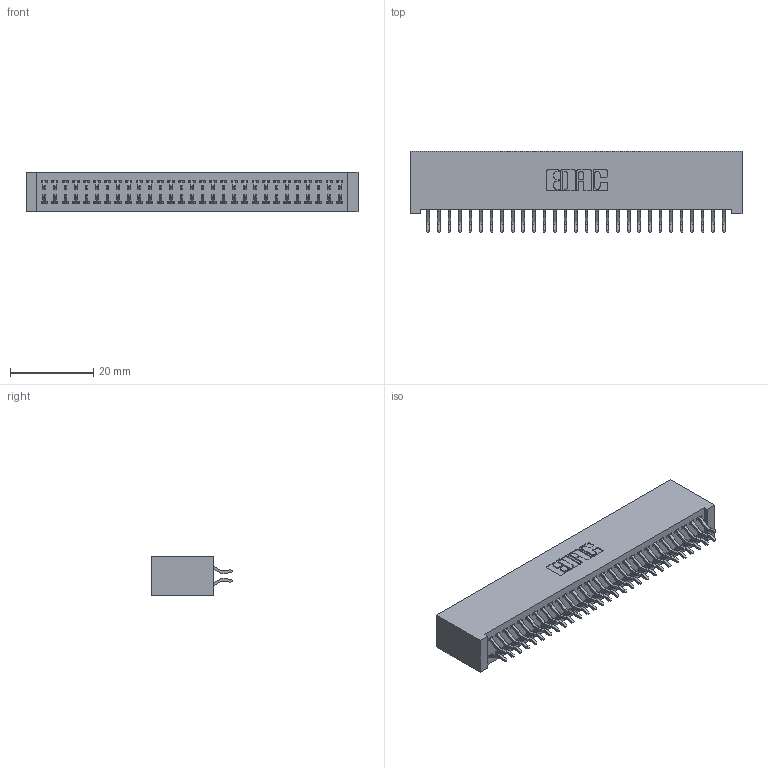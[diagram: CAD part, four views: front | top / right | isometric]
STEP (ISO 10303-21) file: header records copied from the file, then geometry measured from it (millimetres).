
FILE_DESCRIPTION (( 'STEP AP203' ), '1' );
FILE_NAME ('392-058-556-201.STEP', '2019-10-08T16:53:33', ( '' ), ( '' ), 'SwSTEP 2.0', 'SolidWorks 2016', '' );
FILE_SCHEMA (( 'CONFIG_CONTROL_DESIGN' ));
Length unit declared in the file: inch
Products named in the file (3): 392-058-556-201; 342 Part_Lugless; 345-292-001_556 Tail
Assembly tree (59 placements, depth 2):
  392-058-556-201
    342 Part_Lugless
    345-292-001_556 Tail  x58
Bounding box: 79.91 x 19.58 x 9.4 mm (x, y, z)
Volume: 7556.3 mm3; surface area: 12369.3 mm2
Topology: 59 solids, 59 shells, 3466 faces, 10309 edges, 6794 vertices
Faces by surface type: plane 2382, cylinder 1084
Entity records: 20149 total; most frequent: CARTESIAN_POINT 3366, ORIENTED_EDGE 3290, DIRECTION 2881, EDGE_CURVE 1645, VECTOR 1517, LINE 1517, VERTEX_POINT 1094, AXIS2_PLACEMENT_3D 682
